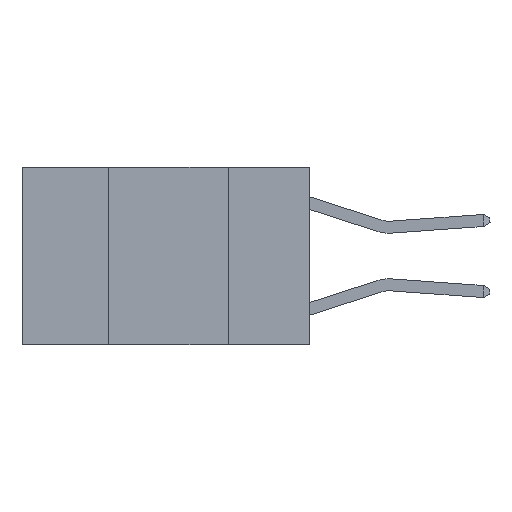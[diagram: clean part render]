
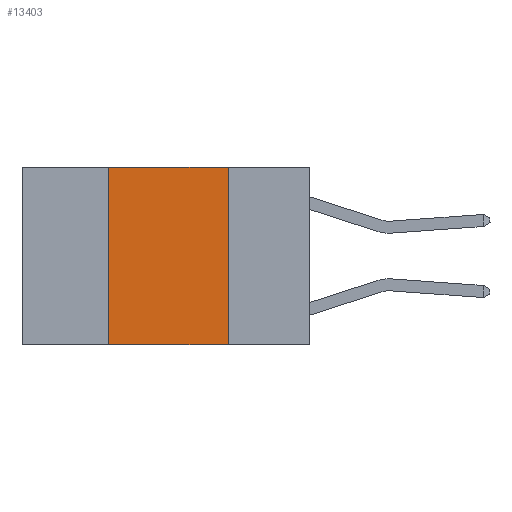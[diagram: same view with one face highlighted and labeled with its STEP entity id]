
A CAD part, left-side view. The second image highlights one B-rep face of the part: STEP entity #13403.
In plain terms, the highlighted planar face has unit normal (-1, 0, 0).
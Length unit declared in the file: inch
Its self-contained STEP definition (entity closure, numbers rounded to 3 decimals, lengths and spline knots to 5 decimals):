
#266 = CARTESIAN_POINT ( 'NONE',  ( 0., 0.6, 0. ) ) ;
#476 = VERTEX_POINT ( 'NONE', #5268 ) ;
#644 = ORIENTED_EDGE ( 'NONE', *, *, #11714, .F. ) ;
#963 = VECTOR ( 'NONE', #4525, 39.37008 ) ;
#1302 = CARTESIAN_POINT ( 'NONE',  ( 0., 0.6, 0. ) ) ;
#1353 = DIRECTION ( 'NONE',  ( 0., 0., -1. ) ) ;
#1488 = CARTESIAN_POINT ( 'NONE',  ( 0., 0.17, -0.37 ) ) ;
#1536 = VECTOR ( 'NONE', #6602, 39.37008 ) ;
#1752 = CARTESIAN_POINT ( 'NONE',  ( 0., 0.17, 0. ) ) ;
#2153 = VERTEX_POINT ( 'NONE', #1488 ) ;
#2201 = FACE_OUTER_BOUND ( 'NONE', #12290, .T. ) ;
#2242 = VECTOR ( 'NONE', #10659, 39.37008 ) ;
#2852 = EDGE_CURVE ( 'NONE', #476, #6378, #3900, .T. ) ;
#3331 = CARTESIAN_POINT ( 'NONE',  ( 0., 0.42, 0. ) ) ;
#3777 = VERTEX_POINT ( 'NONE', #11292 ) ;
#3900 = LINE ( 'NONE', #1302, #963 ) ;
#4200 = ORIENTED_EDGE ( 'NONE', *, *, #11716, .T. ) ;
#4429 = LINE ( 'NONE', #9677, #1536 ) ;
#4525 = DIRECTION ( 'NONE',  ( 0., -1., 0. ) ) ;
#5268 = CARTESIAN_POINT ( 'NONE',  ( 0., 0.42, 0. ) ) ;
#5441 = VECTOR ( 'NONE', #10705, 39.37008 ) ;
#6378 = VERTEX_POINT ( 'NONE', #1752 ) ;
#6602 = DIRECTION ( 'NONE',  ( 0., 0., -1. ) ) ;
#6799 = PLANE ( 'NONE',  #11183 ) ;
#7855 = DIRECTION ( 'NONE',  ( 1., 0., 0. ) ) ;
#7974 = LINE ( 'NONE', #3331, #5441 ) ;
#8300 = LINE ( 'NONE', #8652, #2242 ) ;
#8652 = CARTESIAN_POINT ( 'NONE',  ( 0., 0.6, -0.37 ) ) ;
#9677 = CARTESIAN_POINT ( 'NONE',  ( 0., 0.17, 0. ) ) ;
#10659 = DIRECTION ( 'NONE',  ( 0., -1., 0. ) ) ;
#10705 = DIRECTION ( 'NONE',  ( 0., 0., 1. ) ) ;
#11183 = AXIS2_PLACEMENT_3D ( 'NONE', #266, #7855, #1353 ) ;
#11292 = CARTESIAN_POINT ( 'NONE',  ( 0., 0.42, -0.37 ) ) ;
#11714 = EDGE_CURVE ( 'NONE', #3777, #476, #7974, .T. ) ;
#11716 = EDGE_CURVE ( 'NONE', #3777, #2153, #8300, .T. ) ;
#11754 = EDGE_CURVE ( 'NONE', #6378, #2153, #4429, .T. ) ;
#12290 = EDGE_LOOP ( 'NONE', ( #12385, #12780, #644, #4200 ) ) ;
#12385 = ORIENTED_EDGE ( 'NONE', *, *, #11754, .F. ) ;
#12780 = ORIENTED_EDGE ( 'NONE', *, *, #2852, .F. ) ;
#13403 = ADVANCED_FACE ( 'NONE', ( #2201 ), #6799, .F. ) ;
